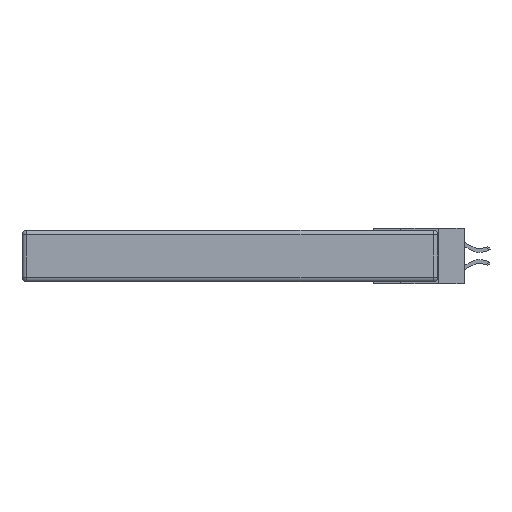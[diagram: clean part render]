
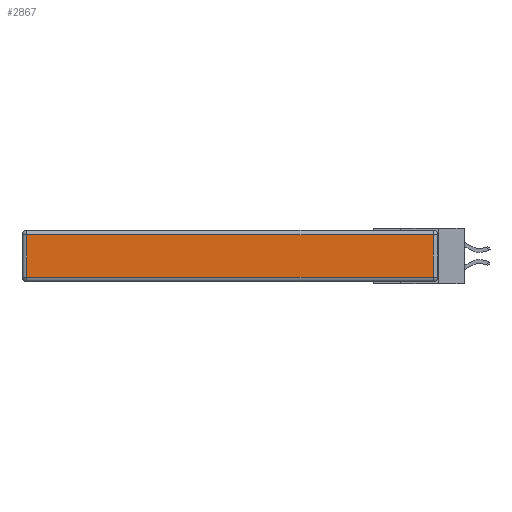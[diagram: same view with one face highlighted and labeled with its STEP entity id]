
A CAD part, left-side view. The second image highlights one B-rep face of the part: STEP entity #2867.
In plain terms, the highlighted planar face has unit normal (-1, 0, 0).
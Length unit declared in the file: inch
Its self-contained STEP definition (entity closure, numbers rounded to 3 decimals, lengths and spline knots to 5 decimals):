
#218 = VECTOR ( 'NONE', #16233, 39.37008 ) ;
#596 = AXIS2_PLACEMENT_3D ( 'NONE', #3178, #5883, #17189 ) ;
#1368 = CARTESIAN_POINT ( 'NONE',  ( 0., 2.75, -0.03 ) ) ;
#1884 = EDGE_CURVE ( 'NONE', #11552, #17290, #9634, .T. ) ;
#2462 = VERTEX_POINT ( 'NONE', #11690 ) ;
#2722 = EDGE_CURVE ( 'NONE', #17290, #13183, #4365, .T. ) ;
#2780 = DIRECTION ( 'NONE',  ( 0., 1., 0. ) ) ;
#2867 = ADVANCED_FACE ( 'NONE', ( #6330 ), #4396, .T. ) ;
#2972 = LINE ( 'NONE', #1368, #12871 ) ;
#3178 = CARTESIAN_POINT ( 'NONE',  ( 0., 0., -0.343 ) ) ;
#3268 = CARTESIAN_POINT ( 'NONE',  ( 0., 2.72, -0.313 ) ) ;
#3340 = CARTESIAN_POINT ( 'NONE',  ( 0., 2.72, -0.343 ) ) ;
#3479 = VECTOR ( 'NONE', #6720, 39.37008 ) ;
#4157 = EDGE_CURVE ( 'NONE', #13183, #2462, #15788, .T. ) ;
#4365 = LINE ( 'NONE', #6547, #3479 ) ;
#4396 = PLANE ( 'NONE',  #596 ) ;
#5751 = EDGE_LOOP ( 'NONE', ( #15830, #6880, #17465, #17740 ) ) ;
#5883 = DIRECTION ( 'NONE',  ( -1., 0., 0. ) ) ;
#6209 = EDGE_CURVE ( 'NONE', #2462, #11552, #2972, .T. ) ;
#6330 = FACE_OUTER_BOUND ( 'NONE', #5751, .T. ) ;
#6547 = CARTESIAN_POINT ( 'NONE',  ( 0., 0., -0.313 ) ) ;
#6720 = DIRECTION ( 'NONE',  ( 0., -1., 0. ) ) ;
#6880 = ORIENTED_EDGE ( 'NONE', *, *, #4157, .T. ) ;
#7123 = CARTESIAN_POINT ( 'NONE',  ( 0., 0.03, -0.313 ) ) ;
#8098 = DIRECTION ( 'NONE',  ( 0., 0., 1. ) ) ;
#9634 = LINE ( 'NONE', #3340, #218 ) ;
#11552 = VERTEX_POINT ( 'NONE', #14657 ) ;
#11690 = CARTESIAN_POINT ( 'NONE',  ( 0., 0.03, -0.03 ) ) ;
#12871 = VECTOR ( 'NONE', #2780, 39.37008 ) ;
#13183 = VERTEX_POINT ( 'NONE', #7123 ) ;
#13355 = VECTOR ( 'NONE', #8098, 39.37008 ) ;
#14657 = CARTESIAN_POINT ( 'NONE',  ( 0., 2.72, -0.03 ) ) ;
#15409 = CARTESIAN_POINT ( 'NONE',  ( 0., 0.03, -0.343 ) ) ;
#15788 = LINE ( 'NONE', #15409, #13355 ) ;
#15830 = ORIENTED_EDGE ( 'NONE', *, *, #2722, .T. ) ;
#16233 = DIRECTION ( 'NONE',  ( 0., 0., -1. ) ) ;
#17189 = DIRECTION ( 'NONE',  ( 0., 0., 1. ) ) ;
#17290 = VERTEX_POINT ( 'NONE', #3268 ) ;
#17465 = ORIENTED_EDGE ( 'NONE', *, *, #6209, .T. ) ;
#17740 = ORIENTED_EDGE ( 'NONE', *, *, #1884, .T. ) ;
